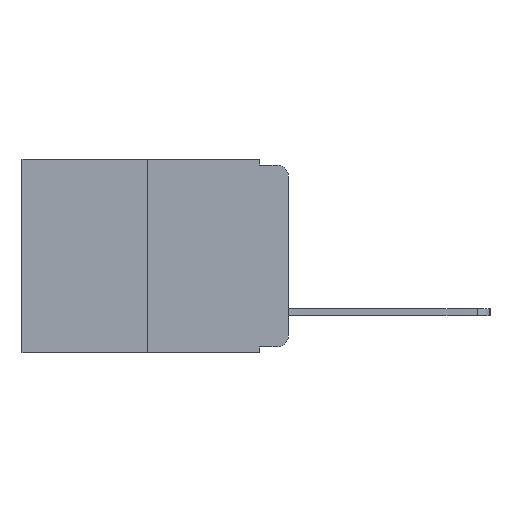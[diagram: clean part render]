
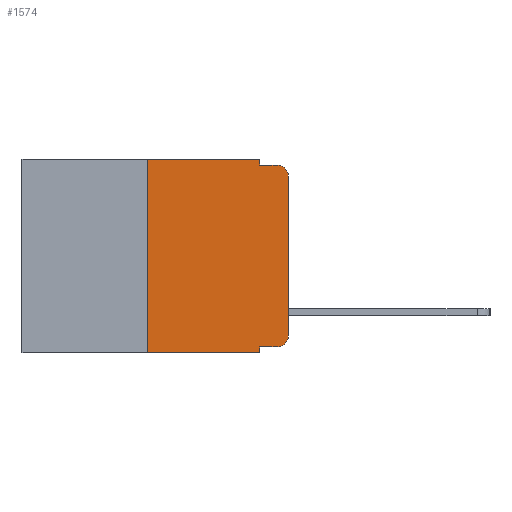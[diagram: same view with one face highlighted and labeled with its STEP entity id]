
A CAD part, left-side view. The second image highlights one B-rep face of the part: STEP entity #1574.
In plain terms, the highlighted planar face has unit normal (-1, 0, 0).
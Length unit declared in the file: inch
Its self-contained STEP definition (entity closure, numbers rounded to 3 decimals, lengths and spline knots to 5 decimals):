
#388 = CARTESIAN_POINT ( 'NONE',  ( 0., 0.051, 0. ) ) ;
#647 = EDGE_CURVE ( 'NONE', #1913, #17539, #15193, .T. ) ;
#1389 = VERTEX_POINT ( 'NONE', #388 ) ;
#1473 = FACE_OUTER_BOUND ( 'NONE', #8454, .T. ) ;
#1574 = ADVANCED_FACE ( 'NONE', ( #1473 ), #18509, .F. ) ;
#1679 = VERTEX_POINT ( 'NONE', #12772 ) ;
#1854 = CARTESIAN_POINT ( 'NONE',  ( 0., 0.02, -0.03 ) ) ;
#1913 = VERTEX_POINT ( 'NONE', #18082 ) ;
#2086 = CARTESIAN_POINT ( 'NONE',  ( 0., 0.051, -0.01 ) ) ;
#2710 = ORIENTED_EDGE ( 'NONE', *, *, #11808, .T. ) ;
#2720 = EDGE_CURVE ( 'NONE', #11310, #1389, #15312, .T. ) ;
#3259 = DIRECTION ( 'NONE',  ( 0., -1., 0. ) ) ;
#3300 = CARTESIAN_POINT ( 'NONE',  ( 0., 0.051, -0.01 ) ) ;
#3434 = AXIS2_PLACEMENT_3D ( 'NONE', #1854, #13157, #3581 ) ;
#3581 = DIRECTION ( 'NONE',  ( 0., 0., -1. ) ) ;
#3721 = ORIENTED_EDGE ( 'NONE', *, *, #5196, .F. ) ;
#3838 = LINE ( 'NONE', #2086, #7621 ) ;
#5116 = LINE ( 'NONE', #6025, #9330 ) ;
#5196 = EDGE_CURVE ( 'NONE', #1679, #11310, #10456, .T. ) ;
#5239 = VERTEX_POINT ( 'NONE', #8561 ) ;
#5723 = VERTEX_POINT ( 'NONE', #14721 ) ;
#6025 = CARTESIAN_POINT ( 'NONE',  ( 0., 0., 0. ) ) ;
#6102 = VERTEX_POINT ( 'NONE', #19108 ) ;
#6202 = DIRECTION ( 'NONE',  ( 0., -1., 0. ) ) ;
#6203 = ORIENTED_EDGE ( 'NONE', *, *, #13742, .T. ) ;
#6707 = VECTOR ( 'NONE', #9945, 39.37008 ) ;
#7591 = AXIS2_PLACEMENT_3D ( 'NONE', #16589, #9348, #12429 ) ;
#7621 = VECTOR ( 'NONE', #18112, 39.37008 ) ;
#7897 = CIRCLE ( 'NONE', #18405, 0.02 ) ;
#7947 = ORIENTED_EDGE ( 'NONE', *, *, #17267, .T. ) ;
#8175 = ORIENTED_EDGE ( 'NONE', *, *, #2720, .F. ) ;
#8408 = EDGE_CURVE ( 'NONE', #1389, #17079, #15337, .T. ) ;
#8454 = EDGE_LOOP ( 'NONE', ( #8768, #6203, #19187, #9899, #8175, #3721, #2710, #18210, #17257, #7947 ) ) ;
#8498 = CARTESIAN_POINT ( 'NONE',  ( 0., 0.25, 0. ) ) ;
#8561 = CARTESIAN_POINT ( 'NONE',  ( 0., 0., -0.03 ) ) ;
#8650 = DIRECTION ( 'NONE',  ( -1., 0., 0. ) ) ;
#8768 = ORIENTED_EDGE ( 'NONE', *, *, #14781, .T. ) ;
#8855 = CARTESIAN_POINT ( 'NONE',  ( 0., 0.25, 0. ) ) ;
#9330 = VECTOR ( 'NONE', #15539, 39.37008 ) ;
#9348 = DIRECTION ( 'NONE',  ( 1., 0., 0. ) ) ;
#9467 = VECTOR ( 'NONE', #19553, 39.37008 ) ;
#9632 = CARTESIAN_POINT ( 'NONE',  ( 0., 0.051, -0.333 ) ) ;
#9899 = ORIENTED_EDGE ( 'NONE', *, *, #8408, .F. ) ;
#9945 = DIRECTION ( 'NONE',  ( 0., 0., -1. ) ) ;
#10062 = VECTOR ( 'NONE', #14566, 39.37008 ) ;
#10456 = LINE ( 'NONE', #8498, #9467 ) ;
#11031 = VERTEX_POINT ( 'NONE', #16090 ) ;
#11038 = CARTESIAN_POINT ( 'NONE',  ( 0., 0.051, 0. ) ) ;
#11226 = VECTOR ( 'NONE', #3259, 39.37008 ) ;
#11310 = VERTEX_POINT ( 'NONE', #8855 ) ;
#11394 = VECTOR ( 'NONE', #13065, 39.37008 ) ;
#11416 = CARTESIAN_POINT ( 'NONE',  ( 0., 0.051, 0. ) ) ;
#11528 = EDGE_CURVE ( 'NONE', #17079, #6102, #3838, .T. ) ;
#11808 = EDGE_CURVE ( 'NONE', #1679, #17539, #15294, .T. ) ;
#11831 = CIRCLE ( 'NONE', #3434, 0.02 ) ;
#12429 = DIRECTION ( 'NONE',  ( 0., 0., -1. ) ) ;
#12486 = CARTESIAN_POINT ( 'NONE',  ( 0., 0.051, -0.343 ) ) ;
#12772 = CARTESIAN_POINT ( 'NONE',  ( 0., 0.25, -0.343 ) ) ;
#13065 = DIRECTION ( 'NONE',  ( 0., 0., -1. ) ) ;
#13157 = DIRECTION ( 'NONE',  ( -1., 0., 0. ) ) ;
#13403 = CARTESIAN_POINT ( 'NONE',  ( 0., 0.473, 0. ) ) ;
#13742 = EDGE_CURVE ( 'NONE', #5239, #6102, #11831, .T. ) ;
#14566 = DIRECTION ( 'NONE',  ( 0., -1., 0. ) ) ;
#14721 = CARTESIAN_POINT ( 'NONE',  ( 0., 0.02, -0.333 ) ) ;
#14781 = EDGE_CURVE ( 'NONE', #11031, #5239, #5116, .T. ) ;
#15193 = LINE ( 'NONE', #11038, #11394 ) ;
#15294 = LINE ( 'NONE', #15708, #18489 ) ;
#15312 = LINE ( 'NONE', #13403, #10062 ) ;
#15337 = LINE ( 'NONE', #11416, #6707 ) ;
#15539 = DIRECTION ( 'NONE',  ( 0., 0., 1. ) ) ;
#15708 = CARTESIAN_POINT ( 'NONE',  ( 0., 0.473, -0.343 ) ) ;
#16090 = CARTESIAN_POINT ( 'NONE',  ( 0., 0., -0.313 ) ) ;
#16589 = CARTESIAN_POINT ( 'NONE',  ( 0., 0.473, 0. ) ) ;
#17079 = VERTEX_POINT ( 'NONE', #3300 ) ;
#17257 = ORIENTED_EDGE ( 'NONE', *, *, #18350, .T. ) ;
#17267 = EDGE_CURVE ( 'NONE', #5723, #11031, #7897, .T. ) ;
#17539 = VERTEX_POINT ( 'NONE', #12486 ) ;
#18082 = CARTESIAN_POINT ( 'NONE',  ( 0., 0.051, -0.333 ) ) ;
#18112 = DIRECTION ( 'NONE',  ( 0., -1., 0. ) ) ;
#18130 = CARTESIAN_POINT ( 'NONE',  ( 0., 0.02, -0.313 ) ) ;
#18210 = ORIENTED_EDGE ( 'NONE', *, *, #647, .F. ) ;
#18350 = EDGE_CURVE ( 'NONE', #1913, #5723, #19677, .T. ) ;
#18405 = AXIS2_PLACEMENT_3D ( 'NONE', #18130, #8650, #19680 ) ;
#18489 = VECTOR ( 'NONE', #6202, 39.37008 ) ;
#18509 = PLANE ( 'NONE',  #7591 ) ;
#19108 = CARTESIAN_POINT ( 'NONE',  ( 0., 0.02, -0.01 ) ) ;
#19187 = ORIENTED_EDGE ( 'NONE', *, *, #11528, .F. ) ;
#19553 = DIRECTION ( 'NONE',  ( 0., 0., 1. ) ) ;
#19677 = LINE ( 'NONE', #9632, #11226 ) ;
#19680 = DIRECTION ( 'NONE',  ( 0., 0., -1. ) ) ;
